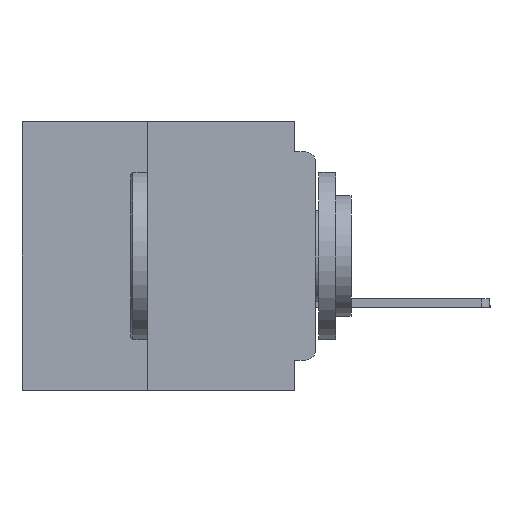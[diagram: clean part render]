
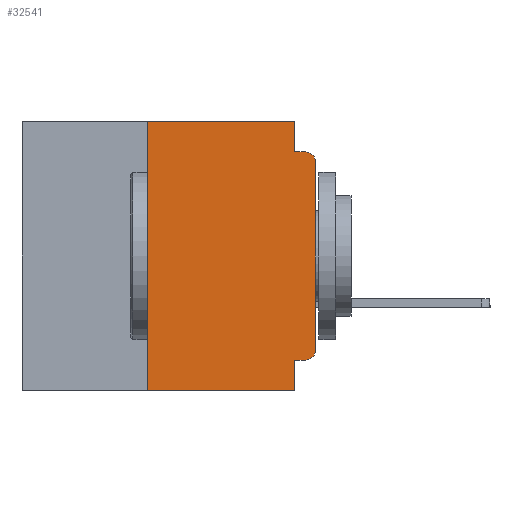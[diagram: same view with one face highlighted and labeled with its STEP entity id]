
A CAD part, left-side view. The second image highlights one B-rep face of the part: STEP entity #32541.
In plain terms, the highlighted planar face has unit normal (-1, 0, 0).
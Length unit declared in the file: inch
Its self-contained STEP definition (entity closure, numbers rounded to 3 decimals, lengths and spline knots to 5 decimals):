
#451 = LINE ( 'NONE', #44833, #50931 ) ;
#768 = DIRECTION ( 'NONE',  ( 0., -1., 0. ) ) ;
#1748 = EDGE_LOOP ( 'NONE', ( #28962, #10860, #5317, #63504, #56533, #44751, #10930, #36982, #51127, #4672 ) ) ;
#2843 = DIRECTION ( 'NONE',  ( 1., 0., 0. ) ) ;
#3283 = EDGE_CURVE ( 'NONE', #44170, #10058, #3348, .T. ) ;
#3348 = CIRCLE ( 'NONE', #10579, 0.015 ) ;
#4672 = ORIENTED_EDGE ( 'NONE', *, *, #39009, .T. ) ;
#5317 = ORIENTED_EDGE ( 'NONE', *, *, #23310, .F. ) ;
#6482 = EDGE_CURVE ( 'NONE', #42309, #30455, #32536, .T. ) ;
#8126 = DIRECTION ( 'NONE',  ( 0., 0., 1. ) ) ;
#9637 = DIRECTION ( 'NONE',  ( 0., -1., 0. ) ) ;
#10058 = VERTEX_POINT ( 'NONE', #27715 ) ;
#10579 = AXIS2_PLACEMENT_3D ( 'NONE', #28055, #27896, #27829 ) ;
#10860 = ORIENTED_EDGE ( 'NONE', *, *, #3283, .T. ) ;
#10930 = ORIENTED_EDGE ( 'NONE', *, *, #19417, .T. ) ;
#13752 = LINE ( 'NONE', #51036, #63944 ) ;
#14730 = CARTESIAN_POINT ( 'NONE',  ( 0., 0.25, 0. ) ) ;
#15566 = FACE_OUTER_BOUND ( 'NONE', #1748, .T. ) ;
#16236 = EDGE_CURVE ( 'NONE', #30455, #49934, #62304, .T. ) ;
#17909 = CARTESIAN_POINT ( 'NONE',  ( 0., 0.437, 0. ) ) ;
#18658 = LINE ( 'NONE', #33315, #30486 ) ;
#19049 = DIRECTION ( 'NONE',  ( 0., 0., -1. ) ) ;
#19161 = VECTOR ( 'NONE', #51478, 39.37008 ) ;
#19417 = EDGE_CURVE ( 'NONE', #50711, #49934, #451, .T. ) ;
#19435 = VERTEX_POINT ( 'NONE', #14730 ) ;
#19891 = CARTESIAN_POINT ( 'NONE',  ( 0., 0.031, 0. ) ) ;
#20452 = EDGE_CURVE ( 'NONE', #50711, #19435, #18658, .T. ) ;
#20566 = DIRECTION ( 'NONE',  ( -1., 0., 0. ) ) ;
#20677 = CARTESIAN_POINT ( 'NONE',  ( 0., 0.437, 0. ) ) ;
#22281 = VECTOR ( 'NONE', #19049, 39.37008 ) ;
#22498 = CARTESIAN_POINT ( 'NONE',  ( 0., 0., -0.34 ) ) ;
#23310 = EDGE_CURVE ( 'NONE', #25017, #10058, #13752, .T. ) ;
#24935 = DIRECTION ( 'NONE',  ( 0., 0., -1. ) ) ;
#25017 = VERTEX_POINT ( 'NONE', #61077 ) ;
#27715 = CARTESIAN_POINT ( 'NONE',  ( 0., 0.015, -0.045 ) ) ;
#27829 = DIRECTION ( 'NONE',  ( 0., 0., -1. ) ) ;
#27896 = DIRECTION ( 'NONE',  ( -1., 0., 0. ) ) ;
#28055 = CARTESIAN_POINT ( 'NONE',  ( 0., 0.015, -0.06 ) ) ;
#28962 = ORIENTED_EDGE ( 'NONE', *, *, #29307, .T. ) ;
#29307 = EDGE_CURVE ( 'NONE', #41003, #44170, #56013, .T. ) ;
#30422 = AXIS2_PLACEMENT_3D ( 'NONE', #50683, #20566, #55709 ) ;
#30455 = VERTEX_POINT ( 'NONE', #36461 ) ;
#30486 = VECTOR ( 'NONE', #58322, 39.37008 ) ;
#32536 = LINE ( 'NONE', #46431, #19161 ) ;
#32541 = ADVANCED_FACE ( 'NONE', ( #15566 ), #33112, .F. ) ;
#33112 = PLANE ( 'NONE',  #35200 ) ;
#33315 = CARTESIAN_POINT ( 'NONE',  ( 0., 0.25, -0.4 ) ) ;
#34465 = EDGE_CURVE ( 'NONE', #52703, #25017, #42933, .T. ) ;
#35200 = AXIS2_PLACEMENT_3D ( 'NONE', #17909, #2843, #38183 ) ;
#35676 = DIRECTION ( 'NONE',  ( 0., -1., 0. ) ) ;
#36461 = CARTESIAN_POINT ( 'NONE',  ( 0., 0.031, -0.355 ) ) ;
#36982 = ORIENTED_EDGE ( 'NONE', *, *, #16236, .F. ) ;
#38183 = DIRECTION ( 'NONE',  ( 0., 0., -1. ) ) ;
#38350 = CARTESIAN_POINT ( 'NONE',  ( 0., 0., 0. ) ) ;
#39009 = EDGE_CURVE ( 'NONE', #42309, #41003, #47429, .T. ) ;
#39851 = VECTOR ( 'NONE', #24935, 39.37008 ) ;
#41003 = VERTEX_POINT ( 'NONE', #22498 ) ;
#42022 = CARTESIAN_POINT ( 'NONE',  ( 0., 0., -0.06 ) ) ;
#42309 = VERTEX_POINT ( 'NONE', #62986 ) ;
#42933 = LINE ( 'NONE', #19891, #39851 ) ;
#43959 = LINE ( 'NONE', #20677, #55732 ) ;
#44084 = CARTESIAN_POINT ( 'NONE',  ( 0., 0.031, -0.4 ) ) ;
#44170 = VERTEX_POINT ( 'NONE', #42022 ) ;
#44751 = ORIENTED_EDGE ( 'NONE', *, *, #20452, .F. ) ;
#44833 = CARTESIAN_POINT ( 'NONE',  ( 0., 0.437, -0.4 ) ) ;
#46431 = CARTESIAN_POINT ( 'NONE',  ( 0., 0., -0.355 ) ) ;
#47429 = CIRCLE ( 'NONE', #30422, 0.015 ) ;
#49934 = VERTEX_POINT ( 'NONE', #55546 ) ;
#50683 = CARTESIAN_POINT ( 'NONE',  ( 0., 0.015, -0.34 ) ) ;
#50711 = VERTEX_POINT ( 'NONE', #62835 ) ;
#50931 = VECTOR ( 'NONE', #9637, 39.37008 ) ;
#51036 = CARTESIAN_POINT ( 'NONE',  ( 0., 0., -0.045 ) ) ;
#51127 = ORIENTED_EDGE ( 'NONE', *, *, #6482, .F. ) ;
#51478 = DIRECTION ( 'NONE',  ( 0., 1., 0. ) ) ;
#52703 = VERTEX_POINT ( 'NONE', #55525 ) ;
#53844 = EDGE_CURVE ( 'NONE', #19435, #52703, #43959, .T. ) ;
#54447 = VECTOR ( 'NONE', #8126, 39.37008 ) ;
#55525 = CARTESIAN_POINT ( 'NONE',  ( 0., 0.031, 0. ) ) ;
#55546 = CARTESIAN_POINT ( 'NONE',  ( 0., 0.031, -0.4 ) ) ;
#55709 = DIRECTION ( 'NONE',  ( 0., 0., -1. ) ) ;
#55732 = VECTOR ( 'NONE', #35676, 39.37008 ) ;
#56013 = LINE ( 'NONE', #38350, #54447 ) ;
#56533 = ORIENTED_EDGE ( 'NONE', *, *, #53844, .F. ) ;
#58322 = DIRECTION ( 'NONE',  ( 0., 0., 1. ) ) ;
#61077 = CARTESIAN_POINT ( 'NONE',  ( 0., 0.031, -0.045 ) ) ;
#62304 = LINE ( 'NONE', #44084, #22281 ) ;
#62835 = CARTESIAN_POINT ( 'NONE',  ( 0., 0.25, -0.4 ) ) ;
#62986 = CARTESIAN_POINT ( 'NONE',  ( 0., 0.015, -0.355 ) ) ;
#63504 = ORIENTED_EDGE ( 'NONE', *, *, #34465, .F. ) ;
#63944 = VECTOR ( 'NONE', #768, 39.37008 ) ;
